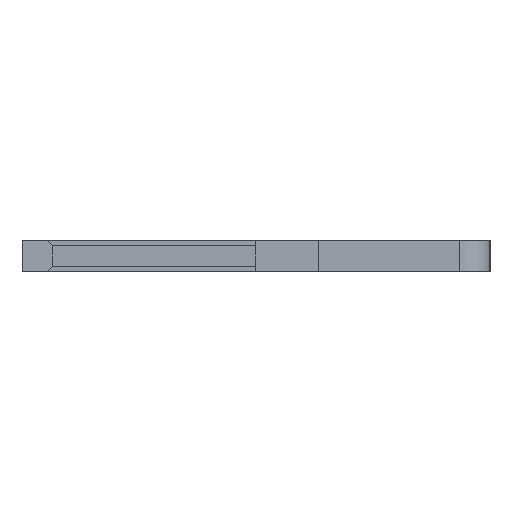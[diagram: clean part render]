
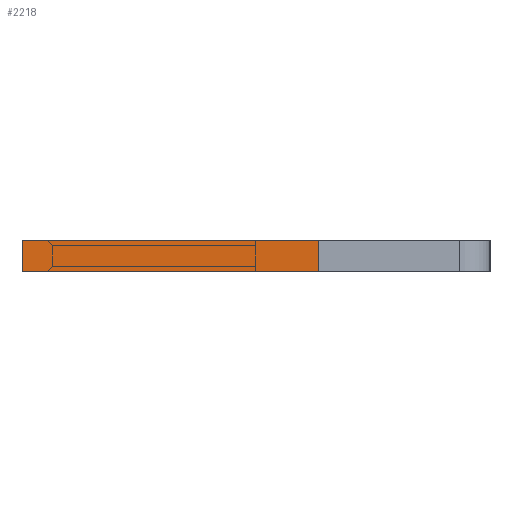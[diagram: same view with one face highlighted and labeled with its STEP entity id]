
A CAD part, left-side view. The second image highlights one B-rep face of the part: STEP entity #2218.
In plain terms, the highlighted face is planar.
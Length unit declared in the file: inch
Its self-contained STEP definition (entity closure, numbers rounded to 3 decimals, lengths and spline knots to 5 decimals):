
#90 = DIRECTION ( 'NONE',  ( -1., 0., 0. ) ) ;
#162 = DIRECTION ( 'NONE',  ( 0., 1., 0. ) ) ;
#175 = DIRECTION ( 'NONE',  ( 1., 0., 0. ) ) ;
#414 = DIRECTION ( 'NONE',  ( 0., 0., 1. ) ) ;
#449 = PLANE ( 'NONE',  #1645 ) ;
#466 = VERTEX_POINT ( 'NONE', #1394 ) ;
#522 = LINE ( 'NONE', #1355, #2716 ) ;
#532 = CARTESIAN_POINT ( 'NONE',  ( 0.01, -0.04, -0.04 ) ) ;
#598 = LINE ( 'NONE', #2875, #2966 ) ;
#782 = EDGE_LOOP ( 'NONE', ( #1154, #2131, #2761, #1670 ) ) ;
#1045 = EDGE_CURVE ( 'NONE', #3065, #2304, #598, .T. ) ;
#1154 = ORIENTED_EDGE ( 'NONE', *, *, #2390, .T. ) ;
#1290 = DIRECTION ( 'NONE',  ( 0., 1., 0. ) ) ;
#1355 = CARTESIAN_POINT ( 'NONE',  ( 0.01, 0.15, -0.04 ) ) ;
#1394 = CARTESIAN_POINT ( 'NONE',  ( -0.01, 0.15, -0.04 ) ) ;
#1645 = AXIS2_PLACEMENT_3D ( 'NONE', #2672, #414, #175 ) ;
#1668 = FACE_OUTER_BOUND ( 'NONE', #782, .T. ) ;
#1670 = ORIENTED_EDGE ( 'NONE', *, *, #1045, .T. ) ;
#1883 = VECTOR ( 'NONE', #162, 39.37008 ) ;
#2014 = VERTEX_POINT ( 'NONE', #3180 ) ;
#2084 = CARTESIAN_POINT ( 'NONE',  ( 0.01, 0.15, -0.04 ) ) ;
#2131 = ORIENTED_EDGE ( 'NONE', *, *, #3441, .F. ) ;
#2179 = VECTOR ( 'NONE', #1290, 39.37008 ) ;
#2218 = ADVANCED_FACE ( 'NONE', ( #1668 ), #449, .F. ) ;
#2304 = VERTEX_POINT ( 'NONE', #3466 ) ;
#2390 = EDGE_CURVE ( 'NONE', #2304, #466, #2917, .T. ) ;
#2423 = EDGE_CURVE ( 'NONE', #3065, #2014, #3353, .T. ) ;
#2672 = CARTESIAN_POINT ( 'NONE',  ( 0.01, 0.15, -0.04 ) ) ;
#2716 = VECTOR ( 'NONE', #90, 39.37008 ) ;
#2761 = ORIENTED_EDGE ( 'NONE', *, *, #2423, .F. ) ;
#2875 = CARTESIAN_POINT ( 'NONE',  ( 0.01, -0.04, -0.04 ) ) ;
#2913 = CARTESIAN_POINT ( 'NONE',  ( -0.01, 0.15, -0.04 ) ) ;
#2917 = LINE ( 'NONE', #2913, #2179 ) ;
#2966 = VECTOR ( 'NONE', #3135, 39.37008 ) ;
#3065 = VERTEX_POINT ( 'NONE', #532 ) ;
#3135 = DIRECTION ( 'NONE',  ( -1., 0., 0. ) ) ;
#3180 = CARTESIAN_POINT ( 'NONE',  ( 0.01, 0.15, -0.04 ) ) ;
#3353 = LINE ( 'NONE', #2084, #1883 ) ;
#3441 = EDGE_CURVE ( 'NONE', #2014, #466, #522, .T. ) ;
#3466 = CARTESIAN_POINT ( 'NONE',  ( -0.01, -0.04, -0.04 ) ) ;
